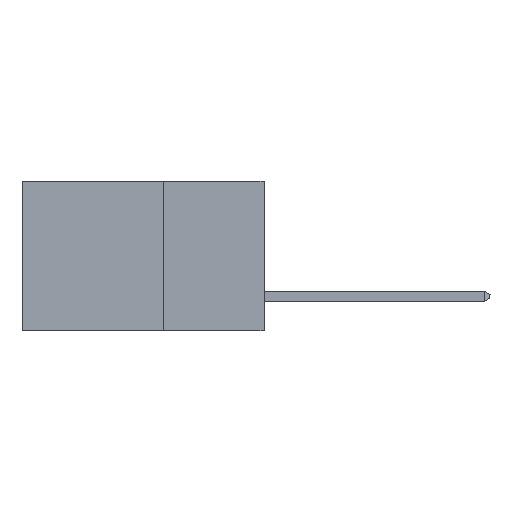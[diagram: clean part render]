
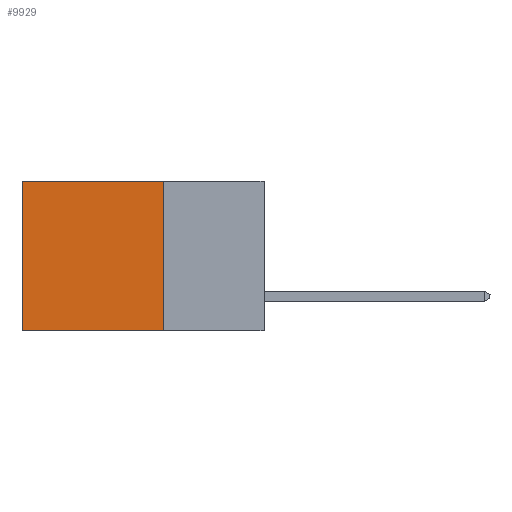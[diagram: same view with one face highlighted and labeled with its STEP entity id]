
A CAD part, left-side view. The second image highlights one B-rep face of the part: STEP entity #9929.
In plain terms, the highlighted planar face has unit normal (-1, 0, 0).
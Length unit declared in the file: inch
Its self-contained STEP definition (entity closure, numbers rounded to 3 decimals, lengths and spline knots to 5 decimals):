
#412 = ORIENTED_EDGE ( 'NONE', *, *, #2795, .F. ) ;
#449 = CARTESIAN_POINT ( 'NONE',  ( 0.2615, 0.25, -0.37 ) ) ;
#515 = VECTOR ( 'NONE', #8301, 39.37008 ) ;
#637 = CARTESIAN_POINT ( 'NONE',  ( 0.2615, 0.6, -0.37 ) ) ;
#1178 = VERTEX_POINT ( 'NONE', #9901 ) ;
#1463 = CARTESIAN_POINT ( 'NONE',  ( 0.2615, 0.25, -0.37 ) ) ;
#1479 = ORIENTED_EDGE ( 'NONE', *, *, #2242, .T. ) ;
#1979 = VERTEX_POINT ( 'NONE', #637 ) ;
#2136 = CARTESIAN_POINT ( 'NONE',  ( 0.2615, 0.25, -0.37 ) ) ;
#2242 = EDGE_CURVE ( 'NONE', #3645, #1979, #6006, .T. ) ;
#2691 = EDGE_LOOP ( 'NONE', ( #1479, #412, #11008, #6698 ) ) ;
#2795 = EDGE_CURVE ( 'NONE', #1178, #1979, #11028, .T. ) ;
#2982 = PLANE ( 'NONE',  #9630 ) ;
#3312 = CARTESIAN_POINT ( 'NONE',  ( 0.2615, 0.25, 0. ) ) ;
#3645 = VERTEX_POINT ( 'NONE', #4787 ) ;
#4139 = VECTOR ( 'NONE', #4275, 39.37008 ) ;
#4275 = DIRECTION ( 'NONE',  ( 0., 0., -1. ) ) ;
#4287 = EDGE_CURVE ( 'NONE', #6888, #3645, #4950, .T. ) ;
#4787 = CARTESIAN_POINT ( 'NONE',  ( 0.2615, 0.6, 0. ) ) ;
#4862 = VECTOR ( 'NONE', #11229, 39.37008 ) ;
#4950 = LINE ( 'NONE', #3312, #5448 ) ;
#5448 = VECTOR ( 'NONE', #10411, 39.37008 ) ;
#5457 = EDGE_CURVE ( 'NONE', #6888, #1178, #10241, .T. ) ;
#5642 = DIRECTION ( 'NONE',  ( 1., 0., 0. ) ) ;
#6006 = LINE ( 'NONE', #8684, #4862 ) ;
#6698 = ORIENTED_EDGE ( 'NONE', *, *, #4287, .T. ) ;
#6888 = VERTEX_POINT ( 'NONE', #7689 ) ;
#7450 = FACE_OUTER_BOUND ( 'NONE', #2691, .T. ) ;
#7689 = CARTESIAN_POINT ( 'NONE',  ( 0.2615, 0.25, 0. ) ) ;
#8301 = DIRECTION ( 'NONE',  ( 0., 1., 0. ) ) ;
#8684 = CARTESIAN_POINT ( 'NONE',  ( 0.2615, 0.6, -0.37 ) ) ;
#9630 = AXIS2_PLACEMENT_3D ( 'NONE', #449, #5642, #10983 ) ;
#9901 = CARTESIAN_POINT ( 'NONE',  ( 0.2615, 0.25, -0.37 ) ) ;
#9929 = ADVANCED_FACE ( 'NONE', ( #7450 ), #2982, .F. ) ;
#10241 = LINE ( 'NONE', #1463, #4139 ) ;
#10411 = DIRECTION ( 'NONE',  ( 0., 1., 0. ) ) ;
#10983 = DIRECTION ( 'NONE',  ( 0., 0., -1. ) ) ;
#11008 = ORIENTED_EDGE ( 'NONE', *, *, #5457, .F. ) ;
#11028 = LINE ( 'NONE', #2136, #515 ) ;
#11229 = DIRECTION ( 'NONE',  ( 0., 0., -1. ) ) ;
